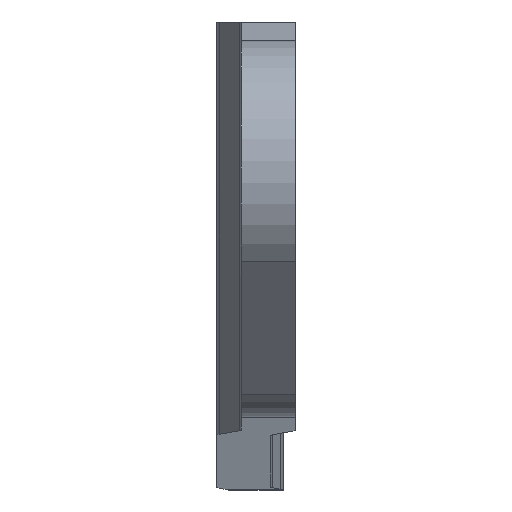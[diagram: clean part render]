
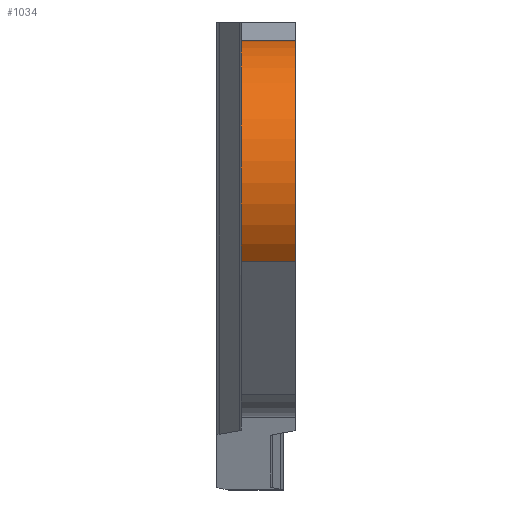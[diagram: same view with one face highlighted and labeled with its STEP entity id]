
A CAD part, top view. The second image highlights one B-rep face of the part: STEP entity #1034.
In plain terms, the highlighted cylindrical face has radius 5.563 mm (diameter 11.125 mm), a partial arc.
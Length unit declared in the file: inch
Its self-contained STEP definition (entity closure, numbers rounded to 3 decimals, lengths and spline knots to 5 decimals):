
#89=FACE_OUTER_BOUND('',#151,.T.);
#151=EDGE_LOOP('',(#804,#805,#806,#807));
#208=CIRCLE('',#1091,0.219);
#213=CIRCLE('',#1111,0.219);
#278=LINE('',#2288,#365);
#292=LINE('',#2331,#379);
#365=VECTOR('',#1236,0.3937);
#379=VECTOR('',#1272,0.3937);
#467=VERTEX_POINT('',#2270);
#468=VERTEX_POINT('',#2272);
#472=VERTEX_POINT('',#2285);
#491=VERTEX_POINT('',#2328);
#575=EDGE_CURVE('',#467,#468,#208,.T.);
#582=EDGE_CURVE('',#472,#467,#278,.T.);
#604=EDGE_CURVE('',#491,#468,#292,.T.);
#607=EDGE_CURVE('',#491,#472,#213,.T.);
#804=ORIENTED_EDGE('',*,*,#607,.F.);
#805=ORIENTED_EDGE('',*,*,#604,.T.);
#806=ORIENTED_EDGE('',*,*,#575,.F.);
#807=ORIENTED_EDGE('',*,*,#582,.F.);
#999=CYLINDRICAL_SURFACE('',#1110,0.219);
#1034=ADVANCED_FACE('',(#89),#999,.T.);
#1091=AXIS2_PLACEMENT_3D('',#2273,#1219,#1220);
#1110=AXIS2_PLACEMENT_3D('',#2336,#1277,#1278);
#1111=AXIS2_PLACEMENT_3D('',#2337,#1279,#1280);
#1219=DIRECTION('center_axis',(-1.,0.,0.));
#1220=DIRECTION('ref_axis',(0.,1.,0.));
#1236=DIRECTION('',(-1.,0.,0.));
#1272=DIRECTION('',(-1.,0.,0.));
#1277=DIRECTION('center_axis',(-1.,0.,0.));
#1278=DIRECTION('ref_axis',(0.,1.,0.));
#1279=DIRECTION('center_axis',(1.,0.,0.));
#1280=DIRECTION('ref_axis',(0.,1.,0.));
#2270=CARTESIAN_POINT('',(-0.55475,-0.39606,3.42818));
#2272=CARTESIAN_POINT('',(-0.55475,-0.031,3.265));
#2273=CARTESIAN_POINT('Origin',(-0.55475,-0.25,3.265));
#2285=CARTESIAN_POINT('',(-0.46475,-0.39606,3.42818));
#2288=CARTESIAN_POINT('',(0.59519,-0.39606,3.42818));
#2328=CARTESIAN_POINT('',(-0.46475,-0.031,3.265));
#2331=CARTESIAN_POINT('',(0.59519,-0.031,3.265));
#2336=CARTESIAN_POINT('Origin',(0.59519,-0.25,3.265));
#2337=CARTESIAN_POINT('Origin',(-0.46475,-0.25,3.265));
